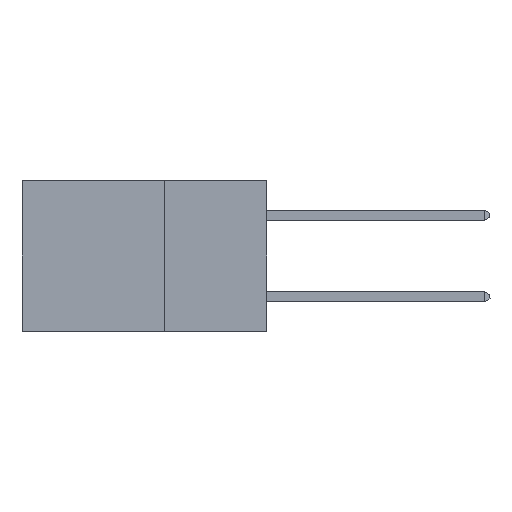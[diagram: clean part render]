
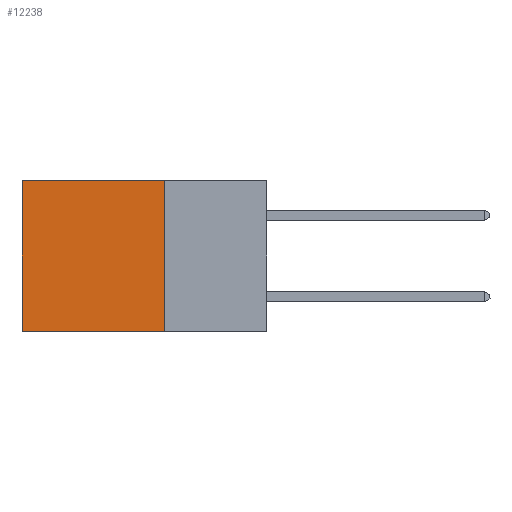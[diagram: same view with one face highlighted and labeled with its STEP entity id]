
A CAD part, left-side view. The second image highlights one B-rep face of the part: STEP entity #12238.
In plain terms, the highlighted planar face has unit normal (-1, 0, 0).
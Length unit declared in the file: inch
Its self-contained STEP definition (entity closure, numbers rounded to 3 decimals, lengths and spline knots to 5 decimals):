
#444 = ORIENTED_EDGE ( 'NONE', *, *, #12952, .T. ) ;
#776 = ORIENTED_EDGE ( 'NONE', *, *, #12361, .F. ) ;
#793 = CARTESIAN_POINT ( 'NONE',  ( 0.2875, 0.6, 0. ) ) ;
#895 = VERTEX_POINT ( 'NONE', #9997 ) ;
#948 = ORIENTED_EDGE ( 'NONE', *, *, #4668, .F. ) ;
#1224 = ORIENTED_EDGE ( 'NONE', *, *, #15355, .T. ) ;
#1722 = DIRECTION ( 'NONE',  ( 0., 1., 0. ) ) ;
#2086 = CARTESIAN_POINT ( 'NONE',  ( 0.2875, 0.6, 0. ) ) ;
#2091 = LINE ( 'NONE', #10069, #6027 ) ;
#2385 = DIRECTION ( 'NONE',  ( 0., 0., -1. ) ) ;
#3249 = LINE ( 'NONE', #793, #10823 ) ;
#4446 = VERTEX_POINT ( 'NONE', #14535 ) ;
#4668 = EDGE_CURVE ( 'NONE', #14506, #895, #12840, .T. ) ;
#4790 = VECTOR ( 'NONE', #15022, 39.37008 ) ;
#6027 = VECTOR ( 'NONE', #6953, 39.37008 ) ;
#6678 = PLANE ( 'NONE',  #17240 ) ;
#6953 = DIRECTION ( 'NONE',  ( 0., 1., 0. ) ) ;
#7197 = VERTEX_POINT ( 'NONE', #2086 ) ;
#8231 = DIRECTION ( 'NONE',  ( 0., 0., -1. ) ) ;
#9118 = CARTESIAN_POINT ( 'NONE',  ( 0.2875, 0.25, 0. ) ) ;
#9997 = CARTESIAN_POINT ( 'NONE',  ( 0.2875, 0.25, -0.37 ) ) ;
#10069 = CARTESIAN_POINT ( 'NONE',  ( 0.2875, 0.25, -0.37 ) ) ;
#10278 = VECTOR ( 'NONE', #1722, 39.37008 ) ;
#10823 = VECTOR ( 'NONE', #2385, 39.37008 ) ;
#12238 = ADVANCED_FACE ( 'NONE', ( #12470 ), #6678, .F. ) ;
#12284 = CARTESIAN_POINT ( 'NONE',  ( 0.2875, 0.25, 0. ) ) ;
#12361 = EDGE_CURVE ( 'NONE', #895, #4446, #2091, .T. ) ;
#12470 = FACE_OUTER_BOUND ( 'NONE', #17682, .T. ) ;
#12840 = LINE ( 'NONE', #9118, #4790 ) ;
#12952 = EDGE_CURVE ( 'NONE', #7197, #4446, #3249, .T. ) ;
#14506 = VERTEX_POINT ( 'NONE', #18974 ) ;
#14535 = CARTESIAN_POINT ( 'NONE',  ( 0.2875, 0.6, -0.37 ) ) ;
#14618 = LINE ( 'NONE', #12284, #10278 ) ;
#15022 = DIRECTION ( 'NONE',  ( 0., 0., -1. ) ) ;
#15355 = EDGE_CURVE ( 'NONE', #14506, #7197, #14618, .T. ) ;
#16946 = CARTESIAN_POINT ( 'NONE',  ( 0.2875, 0.25, 0. ) ) ;
#17016 = DIRECTION ( 'NONE',  ( 1., 0., 0. ) ) ;
#17240 = AXIS2_PLACEMENT_3D ( 'NONE', #16946, #17016, #8231 ) ;
#17682 = EDGE_LOOP ( 'NONE', ( #444, #776, #948, #1224 ) ) ;
#18974 = CARTESIAN_POINT ( 'NONE',  ( 0.2875, 0.25, 0. ) ) ;
